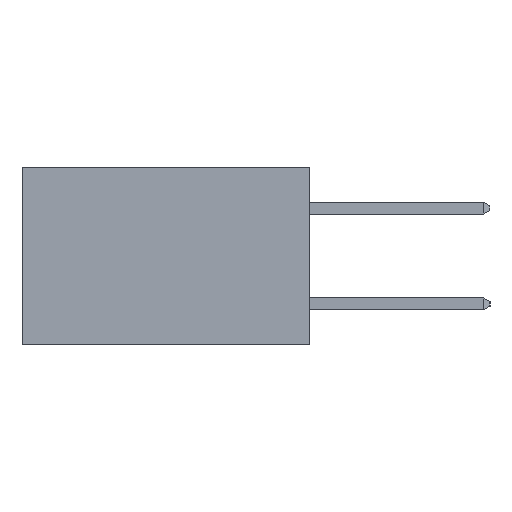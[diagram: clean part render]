
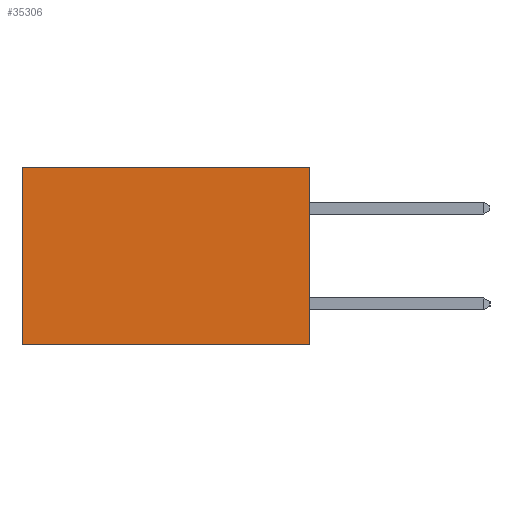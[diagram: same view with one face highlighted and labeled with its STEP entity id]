
A CAD part, left-side view. The second image highlights one B-rep face of the part: STEP entity #35306.
In plain terms, the highlighted planar face has unit normal (-1, 0, 0).
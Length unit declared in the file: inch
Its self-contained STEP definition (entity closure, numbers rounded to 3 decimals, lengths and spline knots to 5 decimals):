
#932 = ORIENTED_EDGE ( 'NONE', *, *, #2194, .T. ) ;
#2194 = EDGE_CURVE ( 'NONE', #3122, #15349, #16836, .T. ) ;
#3122 = VERTEX_POINT ( 'NONE', #6179 ) ;
#4950 = CARTESIAN_POINT ( 'NONE',  ( 0.2875, 0.6, -0.37 ) ) ;
#6179 = CARTESIAN_POINT ( 'NONE',  ( 0.2875, 0., 0. ) ) ;
#6515 = DIRECTION ( 'NONE',  ( 0., 0., -1. ) ) ;
#7146 = DIRECTION ( 'NONE',  ( 0., 0., -1. ) ) ;
#7346 = VERTEX_POINT ( 'NONE', #8427 ) ;
#7758 = PLANE ( 'NONE',  #23776 ) ;
#8427 = CARTESIAN_POINT ( 'NONE',  ( 0.2875, 0., -0.37 ) ) ;
#8504 = LINE ( 'NONE', #29979, #25229 ) ;
#8612 = VECTOR ( 'NONE', #6515, 39.37008 ) ;
#9237 = CARTESIAN_POINT ( 'NONE',  ( 0.2875, 0., 0. ) ) ;
#9694 = CARTESIAN_POINT ( 'NONE',  ( 0.2875, 0.6, 0. ) ) ;
#10126 = FACE_OUTER_BOUND ( 'NONE', #33713, .T. ) ;
#15275 = EDGE_CURVE ( 'NONE', #7346, #34871, #8504, .T. ) ;
#15349 = VERTEX_POINT ( 'NONE', #9694 ) ;
#15530 = ORIENTED_EDGE ( 'NONE', *, *, #28473, .T. ) ;
#15792 = ORIENTED_EDGE ( 'NONE', *, *, #33045, .F. ) ;
#16136 = DIRECTION ( 'NONE',  ( 0., 1., 0. ) ) ;
#16220 = ORIENTED_EDGE ( 'NONE', *, *, #15275, .F. ) ;
#16836 = LINE ( 'NONE', #19734, #34923 ) ;
#17434 = LINE ( 'NONE', #9237, #8612 ) ;
#19734 = CARTESIAN_POINT ( 'NONE',  ( 0.2875, 0., 0. ) ) ;
#20971 = LINE ( 'NONE', #32072, #33362 ) ;
#21958 = DIRECTION ( 'NONE',  ( 1., 0., 0. ) ) ;
#23776 = AXIS2_PLACEMENT_3D ( 'NONE', #32517, #21958, #35591 ) ;
#25229 = VECTOR ( 'NONE', #16136, 39.37008 ) ;
#28473 = EDGE_CURVE ( 'NONE', #15349, #34871, #20971, .T. ) ;
#29979 = CARTESIAN_POINT ( 'NONE',  ( 0.2875, 0., -0.37 ) ) ;
#30848 = DIRECTION ( 'NONE',  ( 0., 1., 0. ) ) ;
#32072 = CARTESIAN_POINT ( 'NONE',  ( 0.2875, 0.6, 0. ) ) ;
#32517 = CARTESIAN_POINT ( 'NONE',  ( 0.2875, 0., 0. ) ) ;
#33045 = EDGE_CURVE ( 'NONE', #3122, #7346, #17434, .T. ) ;
#33362 = VECTOR ( 'NONE', #7146, 39.37008 ) ;
#33713 = EDGE_LOOP ( 'NONE', ( #15530, #16220, #15792, #932 ) ) ;
#34871 = VERTEX_POINT ( 'NONE', #4950 ) ;
#34923 = VECTOR ( 'NONE', #30848, 39.37008 ) ;
#35306 = ADVANCED_FACE ( 'NONE', ( #10126 ), #7758, .F. ) ;
#35591 = DIRECTION ( 'NONE',  ( 0., 0., -1. ) ) ;
